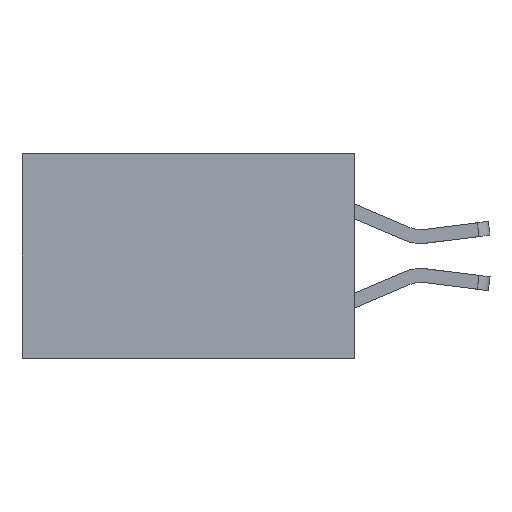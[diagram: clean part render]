
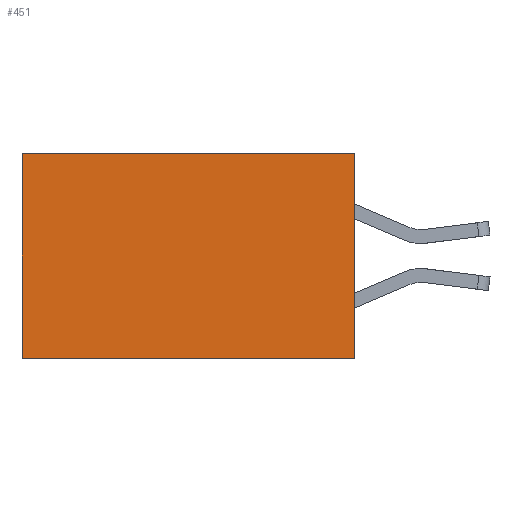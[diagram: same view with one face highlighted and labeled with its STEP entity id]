
A CAD part, left-side view. The second image highlights one B-rep face of the part: STEP entity #451.
In plain terms, the highlighted planar face has unit normal (-1, 0, 0).
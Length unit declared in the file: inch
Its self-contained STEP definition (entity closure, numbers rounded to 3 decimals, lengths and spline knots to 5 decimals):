
#38 = EDGE_CURVE ( 'NONE', #9100, #1899, #7112, .T. ) ;
#326 = LINE ( 'NONE', #7955, #6800 ) ;
#451 = ADVANCED_FACE ( 'NONE', ( #6652 ), #3414, .F. ) ;
#738 = VECTOR ( 'NONE', #7866, 39.37008 ) ;
#1378 = CARTESIAN_POINT ( 'NONE',  ( 0.298, 0.6, -0.37 ) ) ;
#1899 = VERTEX_POINT ( 'NONE', #1378 ) ;
#2002 = VECTOR ( 'NONE', #7670, 39.37008 ) ;
#2040 = CARTESIAN_POINT ( 'NONE',  ( 0.298, 0., 0. ) ) ;
#2519 = ORIENTED_EDGE ( 'NONE', *, *, #38, .T. ) ;
#2622 = VERTEX_POINT ( 'NONE', #4613 ) ;
#2629 = AXIS2_PLACEMENT_3D ( 'NONE', #2040, #7184, #4884 ) ;
#3414 = PLANE ( 'NONE',  #2629 ) ;
#3552 = LINE ( 'NONE', #8743, #3782 ) ;
#3769 = ORIENTED_EDGE ( 'NONE', *, *, #7187, .F. ) ;
#3782 = VECTOR ( 'NONE', #8287, 39.37008 ) ;
#3837 = LINE ( 'NONE', #8387, #2002 ) ;
#4047 = ORIENTED_EDGE ( 'NONE', *, *, #6994, .F. ) ;
#4309 = VERTEX_POINT ( 'NONE', #5388 ) ;
#4569 = EDGE_CURVE ( 'NONE', #4309, #9100, #3552, .T. ) ;
#4613 = CARTESIAN_POINT ( 'NONE',  ( 0.298, 0., -0.37 ) ) ;
#4884 = DIRECTION ( 'NONE',  ( 0., 0., -1. ) ) ;
#4944 = ORIENTED_EDGE ( 'NONE', *, *, #4569, .T. ) ;
#5388 = CARTESIAN_POINT ( 'NONE',  ( 0.298, 0., 0. ) ) ;
#5998 = CARTESIAN_POINT ( 'NONE',  ( 0.298, 0.6, 0. ) ) ;
#6267 = EDGE_LOOP ( 'NONE', ( #2519, #4047, #3769, #4944 ) ) ;
#6652 = FACE_OUTER_BOUND ( 'NONE', #6267, .T. ) ;
#6800 = VECTOR ( 'NONE', #7269, 39.37008 ) ;
#6994 = EDGE_CURVE ( 'NONE', #2622, #1899, #3837, .T. ) ;
#7112 = LINE ( 'NONE', #7133, #738 ) ;
#7133 = CARTESIAN_POINT ( 'NONE',  ( 0.298, 0.6, 0. ) ) ;
#7184 = DIRECTION ( 'NONE',  ( 1., 0., 0. ) ) ;
#7187 = EDGE_CURVE ( 'NONE', #4309, #2622, #326, .T. ) ;
#7269 = DIRECTION ( 'NONE',  ( 0., 0., -1. ) ) ;
#7670 = DIRECTION ( 'NONE',  ( 0., 1., 0. ) ) ;
#7866 = DIRECTION ( 'NONE',  ( 0., 0., -1. ) ) ;
#7955 = CARTESIAN_POINT ( 'NONE',  ( 0.298, 0., 0. ) ) ;
#8287 = DIRECTION ( 'NONE',  ( 0., 1., 0. ) ) ;
#8387 = CARTESIAN_POINT ( 'NONE',  ( 0.298, 0., -0.37 ) ) ;
#8743 = CARTESIAN_POINT ( 'NONE',  ( 0.298, 0., 0. ) ) ;
#9100 = VERTEX_POINT ( 'NONE', #5998 ) ;
